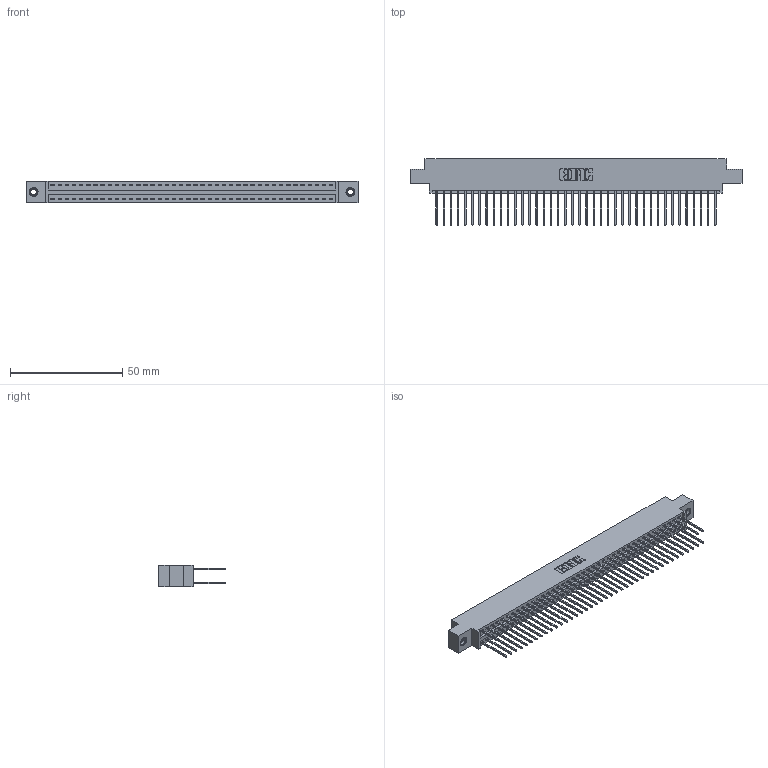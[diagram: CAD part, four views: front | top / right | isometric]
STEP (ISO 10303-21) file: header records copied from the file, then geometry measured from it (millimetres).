
FILE_DESCRIPTION (( 'STEP AP203' ), '1' );
FILE_NAME ('396-080-540-807.STEP', '2018-09-09T20:55:28', ( '' ), ( '' ), 'SwSTEP 2.0', 'SolidWorks 2016', '' );
FILE_SCHEMA (( 'CONFIG_CONTROL_DESIGN' ));
Length unit declared in the file: inch
Products named in the file (4): 345-292-001_345-293-140; 345-250-001_345-250-005-103; 396-080-540-807; 346 Part_0.170 Offset - 0.156 Dia-TI
Assembly tree (83 placements, depth 2):
  396-080-540-807
    346 Part_0.170 Offset - 0.156 Dia-TI
    345-292-001_345-293-140  x80
    345-250-001_345-250-005-103  x2
Bounding box: 147.57 x 29.46 x 9.4 mm (x, y, z)
Volume: 14509.9 mm3; surface area: 21561.3 mm2
Topology: 83 solids, 83 shells, 4346 faces, 12877 edges, 8470 vertices
Faces by surface type: plane 2912, cylinder 1418, cone 12, torus 4
Entity records: 27710 total; most frequent: CARTESIAN_POINT 4555, ORIENTED_EDGE 4482, DIRECTION 4091, EDGE_CURVE 2241, LINE 1929, VECTOR 1929, VERTEX_POINT 1488, AXIS2_PLACEMENT_3D 1081
